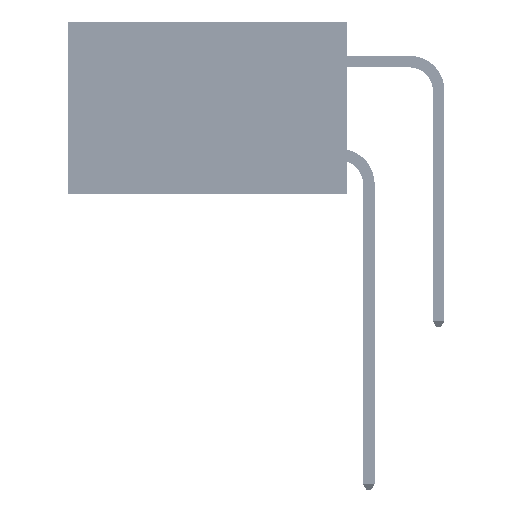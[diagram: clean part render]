
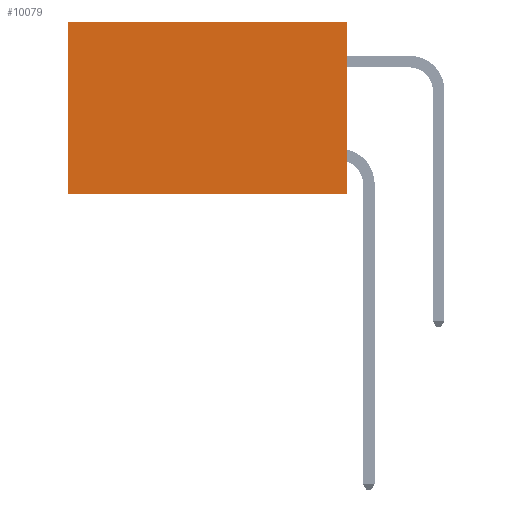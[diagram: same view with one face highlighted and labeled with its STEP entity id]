
A CAD part, left-side view. The second image highlights one B-rep face of the part: STEP entity #10079.
In plain terms, the highlighted planar face has unit normal (-1, 0, 0).
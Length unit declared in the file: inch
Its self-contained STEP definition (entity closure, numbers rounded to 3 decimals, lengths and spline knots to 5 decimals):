
#997 = VECTOR ( 'NONE', #26021, 39.37008 ) ;
#1164 = DIRECTION ( 'NONE',  ( 0., 1., 0. ) ) ;
#6025 = ORIENTED_EDGE ( 'NONE', *, *, #15053, .F. ) ;
#6370 = LINE ( 'NONE', #36614, #15864 ) ;
#6382 = CARTESIAN_POINT ( 'NONE',  ( 0.2875, 0., 0. ) ) ;
#6702 = PLANE ( 'NONE',  #40542 ) ;
#10079 = ADVANCED_FACE ( 'NONE', ( #13930 ), #6702, .F. ) ;
#11384 = CARTESIAN_POINT ( 'NONE',  ( 0.2875, 0., 0. ) ) ;
#13660 = EDGE_CURVE ( 'NONE', #25845, #37339, #42790, .T. ) ;
#13698 = VECTOR ( 'NONE', #41632, 39.37008 ) ;
#13930 = FACE_OUTER_BOUND ( 'NONE', #28906, .T. ) ;
#15053 = EDGE_CURVE ( 'NONE', #16711, #43351, #32129, .T. ) ;
#15113 = CARTESIAN_POINT ( 'NONE',  ( 0.2875, 0., -0.37 ) ) ;
#15864 = VECTOR ( 'NONE', #1164, 39.37008 ) ;
#16711 = VERTEX_POINT ( 'NONE', #6382 ) ;
#17474 = DIRECTION ( 'NONE',  ( 0., 0., -1. ) ) ;
#21060 = CARTESIAN_POINT ( 'NONE',  ( 0.2875, 0., 0. ) ) ;
#23328 = VECTOR ( 'NONE', #41677, 39.37008 ) ;
#24590 = ORIENTED_EDGE ( 'NONE', *, *, #33147, .T. ) ;
#25845 = VERTEX_POINT ( 'NONE', #43997 ) ;
#26021 = DIRECTION ( 'NONE',  ( 0., 0., -1. ) ) ;
#26507 = ORIENTED_EDGE ( 'NONE', *, *, #13660, .T. ) ;
#27807 = CARTESIAN_POINT ( 'NONE',  ( 0.2875, 0.6, 0. ) ) ;
#28906 = EDGE_LOOP ( 'NONE', ( #26507, #45600, #6025, #24590 ) ) ;
#31673 = DIRECTION ( 'NONE',  ( 1., 0., 0. ) ) ;
#31773 = EDGE_CURVE ( 'NONE', #43351, #37339, #34318, .T. ) ;
#32129 = LINE ( 'NONE', #11384, #997 ) ;
#33147 = EDGE_CURVE ( 'NONE', #16711, #25845, #6370, .T. ) ;
#34318 = LINE ( 'NONE', #38348, #13698 ) ;
#36614 = CARTESIAN_POINT ( 'NONE',  ( 0.2875, 0., 0. ) ) ;
#37339 = VERTEX_POINT ( 'NONE', #41555 ) ;
#38348 = CARTESIAN_POINT ( 'NONE',  ( 0.2875, 0., -0.37 ) ) ;
#40542 = AXIS2_PLACEMENT_3D ( 'NONE', #21060, #31673, #17474 ) ;
#41555 = CARTESIAN_POINT ( 'NONE',  ( 0.2875, 0.6, -0.37 ) ) ;
#41632 = DIRECTION ( 'NONE',  ( 0., 1., 0. ) ) ;
#41677 = DIRECTION ( 'NONE',  ( 0., 0., -1. ) ) ;
#42790 = LINE ( 'NONE', #27807, #23328 ) ;
#43351 = VERTEX_POINT ( 'NONE', #15113 ) ;
#43997 = CARTESIAN_POINT ( 'NONE',  ( 0.2875, 0.6, 0. ) ) ;
#45600 = ORIENTED_EDGE ( 'NONE', *, *, #31773, .F. ) ;
